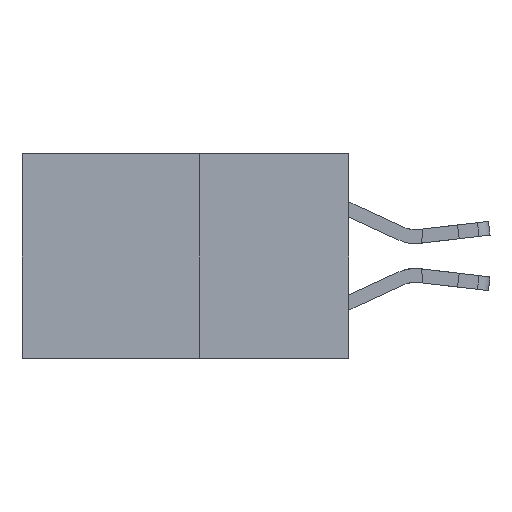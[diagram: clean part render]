
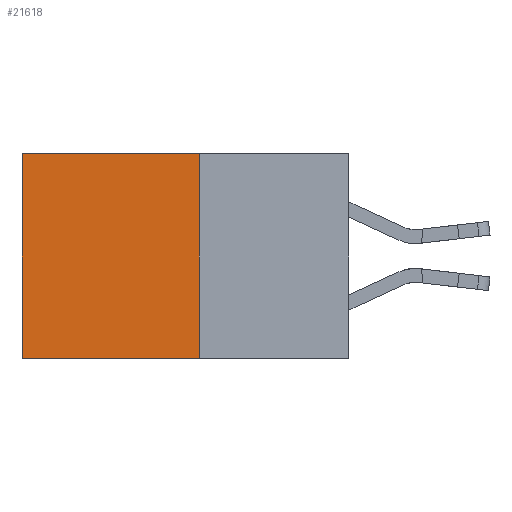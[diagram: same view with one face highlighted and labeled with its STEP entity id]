
A CAD part, left-side view. The second image highlights one B-rep face of the part: STEP entity #21618.
In plain terms, the highlighted planar face has unit normal (-1, 0, 0).
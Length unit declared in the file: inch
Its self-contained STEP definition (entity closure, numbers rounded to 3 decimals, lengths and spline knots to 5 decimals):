
#114 = EDGE_CURVE ( 'NONE', #29197, #25997, #3375, .T. ) ;
#1078 = DIRECTION ( 'NONE',  ( 0., 1., 0. ) ) ;
#2840 = CARTESIAN_POINT ( 'NONE',  ( 0.277, 0.27, -0.37 ) ) ;
#3375 = LINE ( 'NONE', #28446, #4106 ) ;
#3764 = DIRECTION ( 'NONE',  ( 0., 0., -1. ) ) ;
#4007 = CARTESIAN_POINT ( 'NONE',  ( 0.277, 0.27, -0.37 ) ) ;
#4106 = VECTOR ( 'NONE', #28548, 39.37008 ) ;
#4629 = CARTESIAN_POINT ( 'NONE',  ( 0.277, 0.59, -0.37 ) ) ;
#5028 = FACE_OUTER_BOUND ( 'NONE', #27415, .T. ) ;
#5124 = LINE ( 'NONE', #2840, #17458 ) ;
#6415 = EDGE_CURVE ( 'NONE', #25997, #9748, #16413, .T. ) ;
#6980 = DIRECTION ( 'NONE',  ( 0., 0., -1. ) ) ;
#9208 = ORIENTED_EDGE ( 'NONE', *, *, #6415, .T. ) ;
#9573 = EDGE_CURVE ( 'NONE', #29197, #26079, #5124, .T. ) ;
#9748 = VERTEX_POINT ( 'NONE', #24186 ) ;
#10276 = VECTOR ( 'NONE', #6980, 39.37008 ) ;
#13031 = CARTESIAN_POINT ( 'NONE',  ( 0.277, 0.27, -0.37 ) ) ;
#13993 = ORIENTED_EDGE ( 'NONE', *, *, #9573, .F. ) ;
#15346 = PLANE ( 'NONE',  #27085 ) ;
#15387 = CARTESIAN_POINT ( 'NONE',  ( 0.277, 0.59, 0. ) ) ;
#16413 = LINE ( 'NONE', #4629, #10276 ) ;
#17458 = VECTOR ( 'NONE', #19050, 39.37008 ) ;
#17646 = DIRECTION ( 'NONE',  ( 1., 0., 0. ) ) ;
#18010 = EDGE_CURVE ( 'NONE', #26079, #9748, #20403, .T. ) ;
#19050 = DIRECTION ( 'NONE',  ( 0., 0., -1. ) ) ;
#19687 = VECTOR ( 'NONE', #1078, 39.37008 ) ;
#20403 = LINE ( 'NONE', #21927, #19687 ) ;
#21618 = ADVANCED_FACE ( 'NONE', ( #5028 ), #15346, .F. ) ;
#21927 = CARTESIAN_POINT ( 'NONE',  ( 0.277, 0.27, -0.37 ) ) ;
#24064 = CARTESIAN_POINT ( 'NONE',  ( 0.277, 0.27, 0. ) ) ;
#24186 = CARTESIAN_POINT ( 'NONE',  ( 0.277, 0.59, -0.37 ) ) ;
#25997 = VERTEX_POINT ( 'NONE', #15387 ) ;
#26079 = VERTEX_POINT ( 'NONE', #4007 ) ;
#27085 = AXIS2_PLACEMENT_3D ( 'NONE', #13031, #17646, #3764 ) ;
#27415 = EDGE_LOOP ( 'NONE', ( #9208, #27980, #13993, #27593 ) ) ;
#27593 = ORIENTED_EDGE ( 'NONE', *, *, #114, .T. ) ;
#27980 = ORIENTED_EDGE ( 'NONE', *, *, #18010, .F. ) ;
#28446 = CARTESIAN_POINT ( 'NONE',  ( 0.277, 0.27, 0. ) ) ;
#28548 = DIRECTION ( 'NONE',  ( 0., 1., 0. ) ) ;
#29197 = VERTEX_POINT ( 'NONE', #24064 ) ;
